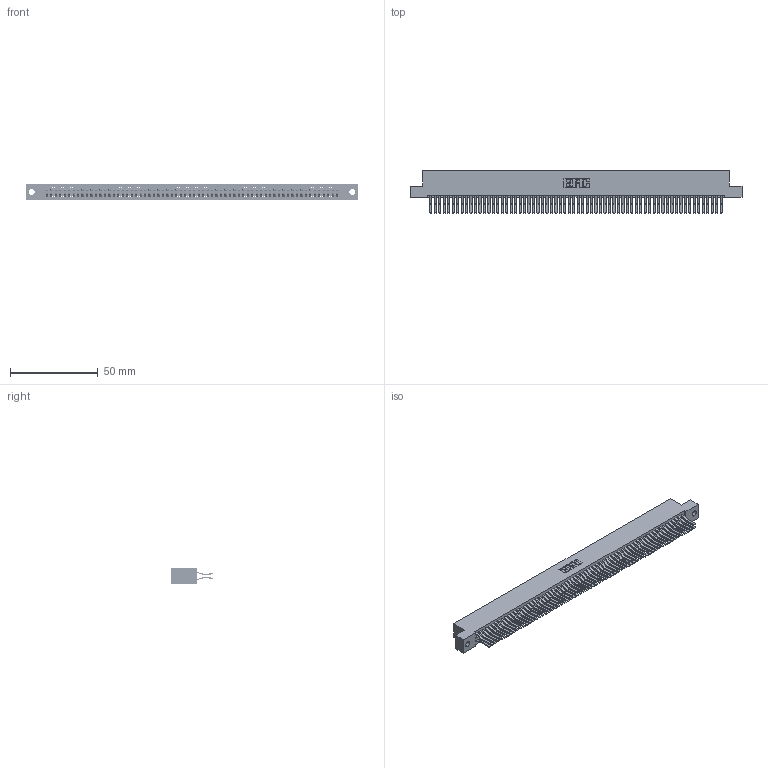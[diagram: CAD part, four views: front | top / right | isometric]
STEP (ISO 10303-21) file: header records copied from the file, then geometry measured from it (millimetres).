
FILE_DESCRIPTION (( 'STEP AP203' ), '1' );
FILE_NAME ('395-132-560-202.STEP', '2019-10-29T08:18:13', ( '' ), ( '' ), 'SwSTEP 2.0', 'SolidWorks 2016', '' );
FILE_SCHEMA (( 'CONFIG_CONTROL_DESIGN' ));
Length unit declared in the file: inch
Products named in the file (3): 345 Part_Flush Mounting Lugs - 0.128 Dia; 345-292-001_560 Tail; 395-132-560-202
Assembly tree (133 placements, depth 2):
  395-132-560-202
    345 Part_Flush Mounting Lugs - 0.128 Dia
    345-292-001_560 Tail  x132
Bounding box: 188.85 x 24.45 x 9.4 mm (x, y, z)
Volume: 19396.3 mm3; surface area: 31088.3 mm2
Topology: 133 solids, 133 shells, 6990 faces, 20801 edges, 13690 vertices
Faces by surface type: plane 4436, cylinder 2554
Entity records: 48645 total; most frequent: CARTESIAN_POINT 8132, ORIENTED_EDGE 8066, DIRECTION 7145, EDGE_CURVE 4033, VECTOR 3633, LINE 3633, VERTEX_POINT 2686, AXIS2_PLACEMENT_3D 1756
